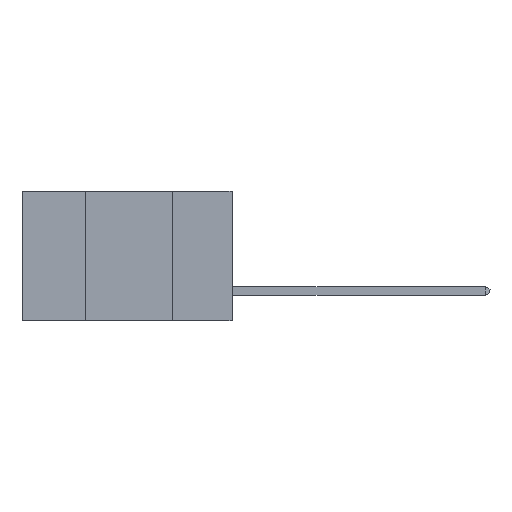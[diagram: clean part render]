
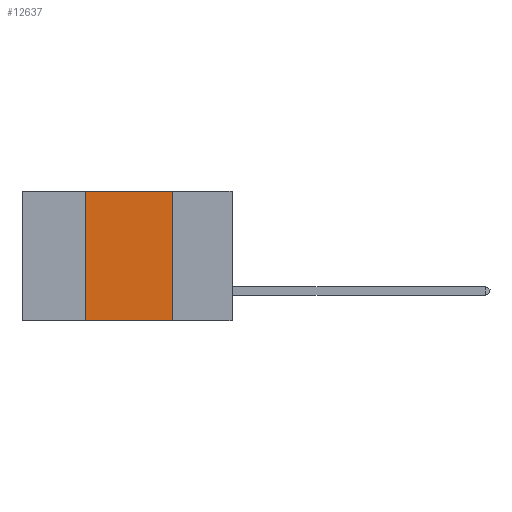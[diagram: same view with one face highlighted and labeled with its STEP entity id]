
A CAD part, left-side view. The second image highlights one B-rep face of the part: STEP entity #12637.
In plain terms, the highlighted planar face has unit normal (-1, 0, 0).
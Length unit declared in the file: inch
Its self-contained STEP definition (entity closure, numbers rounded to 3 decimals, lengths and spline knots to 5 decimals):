
#175 = VERTEX_POINT ( 'NONE', #3265 ) ;
#354 = VECTOR ( 'NONE', #3899, 39.37008 ) ;
#378 = CARTESIAN_POINT ( 'NONE',  ( 0., 0.42, 0. ) ) ;
#857 = ORIENTED_EDGE ( 'NONE', *, *, #11741, .T. ) ;
#1089 = DIRECTION ( 'NONE',  ( 0., 0., 1. ) ) ;
#1469 = EDGE_CURVE ( 'NONE', #7599, #6426, #3370, .T. ) ;
#1485 = EDGE_LOOP ( 'NONE', ( #10234, #4109, #7793, #857 ) ) ;
#2717 = AXIS2_PLACEMENT_3D ( 'NONE', #10824, #6537, #6446 ) ;
#2786 = CARTESIAN_POINT ( 'NONE',  ( 0., 0.17, 0. ) ) ;
#3066 = CARTESIAN_POINT ( 'NONE',  ( 0., 0.17, -0.37 ) ) ;
#3194 = EDGE_CURVE ( 'NONE', #6426, #13732, #5160, .T. ) ;
#3197 = LINE ( 'NONE', #8088, #10853 ) ;
#3265 = CARTESIAN_POINT ( 'NONE',  ( 0., 0.42, -0.37 ) ) ;
#3351 = LINE ( 'NONE', #3358, #4675 ) ;
#3358 = CARTESIAN_POINT ( 'NONE',  ( 0., 0.42, 0. ) ) ;
#3370 = LINE ( 'NONE', #12934, #12356 ) ;
#3899 = DIRECTION ( 'NONE',  ( 0., 0., -1. ) ) ;
#4109 = ORIENTED_EDGE ( 'NONE', *, *, #1469, .F. ) ;
#4675 = VECTOR ( 'NONE', #1089, 39.37008 ) ;
#5160 = LINE ( 'NONE', #2786, #354 ) ;
#5771 = CARTESIAN_POINT ( 'NONE',  ( 0., 0.17, 0. ) ) ;
#6426 = VERTEX_POINT ( 'NONE', #5771 ) ;
#6446 = DIRECTION ( 'NONE',  ( 0., 0., -1. ) ) ;
#6519 = DIRECTION ( 'NONE',  ( 0., -1., 0. ) ) ;
#6537 = DIRECTION ( 'NONE',  ( 1., 0., 0. ) ) ;
#7599 = VERTEX_POINT ( 'NONE', #378 ) ;
#7793 = ORIENTED_EDGE ( 'NONE', *, *, #11937, .F. ) ;
#8088 = CARTESIAN_POINT ( 'NONE',  ( 0., 0.6, -0.37 ) ) ;
#9986 = FACE_OUTER_BOUND ( 'NONE', #1485, .T. ) ;
#10234 = ORIENTED_EDGE ( 'NONE', *, *, #3194, .F. ) ;
#10321 = DIRECTION ( 'NONE',  ( 0., -1., 0. ) ) ;
#10824 = CARTESIAN_POINT ( 'NONE',  ( 0., 0.6, 0. ) ) ;
#10853 = VECTOR ( 'NONE', #10321, 39.37008 ) ;
#11741 = EDGE_CURVE ( 'NONE', #175, #13732, #3197, .T. ) ;
#11903 = PLANE ( 'NONE',  #2717 ) ;
#11937 = EDGE_CURVE ( 'NONE', #175, #7599, #3351, .T. ) ;
#12356 = VECTOR ( 'NONE', #6519, 39.37008 ) ;
#12637 = ADVANCED_FACE ( 'NONE', ( #9986 ), #11903, .F. ) ;
#12934 = CARTESIAN_POINT ( 'NONE',  ( 0., 0.6, 0. ) ) ;
#13732 = VERTEX_POINT ( 'NONE', #3066 ) ;
